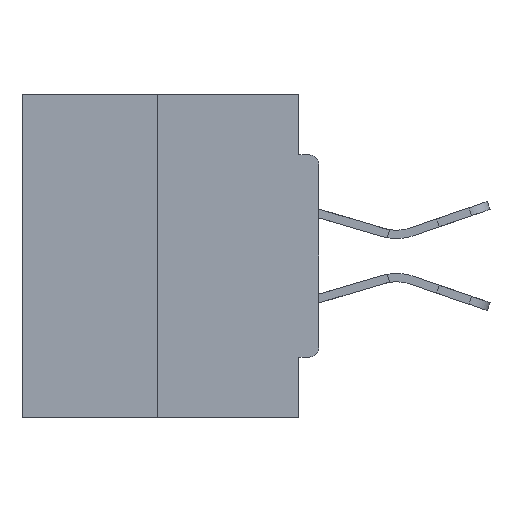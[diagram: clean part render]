
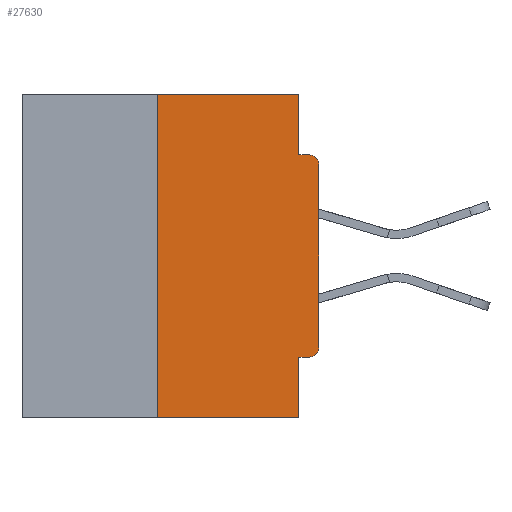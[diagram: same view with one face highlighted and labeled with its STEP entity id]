
A CAD part, left-side view. The second image highlights one B-rep face of the part: STEP entity #27630.
In plain terms, the highlighted planar face has unit normal (-1, 0, 0).
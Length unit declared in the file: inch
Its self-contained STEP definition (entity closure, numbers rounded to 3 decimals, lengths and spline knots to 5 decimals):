
#457 = CARTESIAN_POINT ( 'NONE',  ( 0., 0.46, 0. ) ) ;
#1142 = CARTESIAN_POINT ( 'NONE',  ( 0., 0., -0.3915 ) ) ;
#1156 = AXIS2_PLACEMENT_3D ( 'NONE', #34447, #14426, #34710 ) ;
#1376 = VECTOR ( 'NONE', #11448, 39.37008 ) ;
#2702 = VECTOR ( 'NONE', #17918, 39.37008 ) ;
#3242 = PLANE ( 'NONE',  #1156 ) ;
#3441 = CARTESIAN_POINT ( 'NONE',  ( 0., 0.031, 0. ) ) ;
#3886 = ORIENTED_EDGE ( 'NONE', *, *, #33453, .T. ) ;
#4146 = LINE ( 'NONE', #34895, #21354 ) ;
#4698 = LINE ( 'NONE', #6430, #34525 ) ;
#4746 = EDGE_LOOP ( 'NONE', ( #10892, #16210, #3886, #9443, #21382, #37385, #18964, #7743, #18759, #13536 ) ) ;
#5447 = VERTEX_POINT ( 'NONE', #27406 ) ;
#5451 = VERTEX_POINT ( 'NONE', #23495 ) ;
#5515 = DIRECTION ( 'NONE',  ( 0., -1., 0. ) ) ;
#5622 = CARTESIAN_POINT ( 'NONE',  ( 0., 0.015, -0.3915 ) ) ;
#6350 = VECTOR ( 'NONE', #9418, 39.37008 ) ;
#6430 = CARTESIAN_POINT ( 'NONE',  ( 0., 0.031, -0.5 ) ) ;
#7446 = EDGE_CURVE ( 'NONE', #5451, #9716, #4146, .T. ) ;
#7743 = ORIENTED_EDGE ( 'NONE', *, *, #12546, .T. ) ;
#8272 = CARTESIAN_POINT ( 'NONE',  ( 0., 0.031, 0. ) ) ;
#8550 = DIRECTION ( 'NONE',  ( 0., 0., -1. ) ) ;
#8552 = EDGE_CURVE ( 'NONE', #5447, #15284, #35614, .T. ) ;
#8675 = CARTESIAN_POINT ( 'NONE',  ( 0., 0., -0.0935 ) ) ;
#9080 = LINE ( 'NONE', #22779, #1376 ) ;
#9205 = DIRECTION ( 'NONE',  ( 0., -1., 0. ) ) ;
#9327 = AXIS2_PLACEMENT_3D ( 'NONE', #5622, #25803, #8550 ) ;
#9418 = DIRECTION ( 'NONE',  ( 0., 1., 0. ) ) ;
#9443 = ORIENTED_EDGE ( 'NONE', *, *, #31151, .F. ) ;
#9617 = DIRECTION ( 'NONE',  ( -1., 0., 0. ) ) ;
#9716 = VERTEX_POINT ( 'NONE', #27413 ) ;
#10869 = CARTESIAN_POINT ( 'NONE',  ( 0., 0.015, -0.0935 ) ) ;
#10892 = ORIENTED_EDGE ( 'NONE', *, *, #35141, .F. ) ;
#11448 = DIRECTION ( 'NONE',  ( 0., -1., 0. ) ) ;
#12361 = CARTESIAN_POINT ( 'NONE',  ( 0., 0., 0. ) ) ;
#12546 = EDGE_CURVE ( 'NONE', #15391, #25123, #28562, .T. ) ;
#13536 = ORIENTED_EDGE ( 'NONE', *, *, #34450, .F. ) ;
#13835 = VECTOR ( 'NONE', #5515, 39.37008 ) ;
#14426 = DIRECTION ( 'NONE',  ( 1., 0., 0. ) ) ;
#14613 = DIRECTION ( 'NONE',  ( 0., 0., -1. ) ) ;
#14791 = VERTEX_POINT ( 'NONE', #23134 ) ;
#14971 = LINE ( 'NONE', #8272, #29389 ) ;
#15254 = CARTESIAN_POINT ( 'NONE',  ( 0., 0., -0.4065 ) ) ;
#15284 = VERTEX_POINT ( 'NONE', #1142 ) ;
#15333 = CARTESIAN_POINT ( 'NONE',  ( 0., 0.015, -0.1085 ) ) ;
#15391 = VERTEX_POINT ( 'NONE', #18413 ) ;
#16210 = ORIENTED_EDGE ( 'NONE', *, *, #7446, .F. ) ;
#16266 = FACE_OUTER_BOUND ( 'NONE', #4746, .T. ) ;
#16281 = CARTESIAN_POINT ( 'NONE',  ( 0., 0.031, -0.4065 ) ) ;
#17630 = DIRECTION ( 'NONE',  ( 0., 0., 1. ) ) ;
#17918 = DIRECTION ( 'NONE',  ( 0., 0., 1. ) ) ;
#18413 = CARTESIAN_POINT ( 'NONE',  ( 0., 0., -0.1085 ) ) ;
#18759 = ORIENTED_EDGE ( 'NONE', *, *, #21937, .F. ) ;
#18964 = ORIENTED_EDGE ( 'NONE', *, *, #25214, .T. ) ;
#19540 = AXIS2_PLACEMENT_3D ( 'NONE', #15333, #9617, #27264 ) ;
#21354 = VECTOR ( 'NONE', #17630, 39.37008 ) ;
#21382 = ORIENTED_EDGE ( 'NONE', *, *, #27041, .F. ) ;
#21692 = LINE ( 'NONE', #15254, #6350 ) ;
#21937 = EDGE_CURVE ( 'NONE', #36674, #25123, #24209, .T. ) ;
#22779 = CARTESIAN_POINT ( 'NONE',  ( 0., 0.46, -0.5 ) ) ;
#23134 = CARTESIAN_POINT ( 'NONE',  ( 0., 0.031, -0.5 ) ) ;
#23495 = CARTESIAN_POINT ( 'NONE',  ( 0., 0.25, -0.5 ) ) ;
#24209 = LINE ( 'NONE', #8675, #13835 ) ;
#24739 = VECTOR ( 'NONE', #9205, 39.37008 ) ;
#25123 = VERTEX_POINT ( 'NONE', #10869 ) ;
#25214 = EDGE_CURVE ( 'NONE', #15284, #15391, #35257, .T. ) ;
#25803 = DIRECTION ( 'NONE',  ( -1., 0., 0. ) ) ;
#27041 = EDGE_CURVE ( 'NONE', #5447, #27745, #21692, .T. ) ;
#27264 = DIRECTION ( 'NONE',  ( 0., 0., -1. ) ) ;
#27406 = CARTESIAN_POINT ( 'NONE',  ( 0., 0.015, -0.4065 ) ) ;
#27413 = CARTESIAN_POINT ( 'NONE',  ( 0., 0.25, 0. ) ) ;
#27630 = ADVANCED_FACE ( 'NONE', ( #16266 ), #3242, .F. ) ;
#27745 = VERTEX_POINT ( 'NONE', #16281 ) ;
#28562 = CIRCLE ( 'NONE', #19540, 0.015 ) ;
#29389 = VECTOR ( 'NONE', #14613, 39.37008 ) ;
#31151 = EDGE_CURVE ( 'NONE', #27745, #14791, #4698, .T. ) ;
#32325 = DIRECTION ( 'NONE',  ( 0., 0., -1. ) ) ;
#33453 = EDGE_CURVE ( 'NONE', #5451, #14791, #9080, .T. ) ;
#34447 = CARTESIAN_POINT ( 'NONE',  ( 0., 0.46, 0. ) ) ;
#34450 = EDGE_CURVE ( 'NONE', #36867, #36674, #14971, .T. ) ;
#34525 = VECTOR ( 'NONE', #32325, 39.37008 ) ;
#34710 = DIRECTION ( 'NONE',  ( 0., 0., -1. ) ) ;
#34895 = CARTESIAN_POINT ( 'NONE',  ( 0., 0.25, 0. ) ) ;
#35141 = EDGE_CURVE ( 'NONE', #9716, #36867, #37412, .T. ) ;
#35257 = LINE ( 'NONE', #12361, #2702 ) ;
#35473 = CARTESIAN_POINT ( 'NONE',  ( 0., 0.031, -0.0935 ) ) ;
#35614 = CIRCLE ( 'NONE', #9327, 0.015 ) ;
#36674 = VERTEX_POINT ( 'NONE', #35473 ) ;
#36867 = VERTEX_POINT ( 'NONE', #3441 ) ;
#37385 = ORIENTED_EDGE ( 'NONE', *, *, #8552, .T. ) ;
#37412 = LINE ( 'NONE', #457, #24739 ) ;
